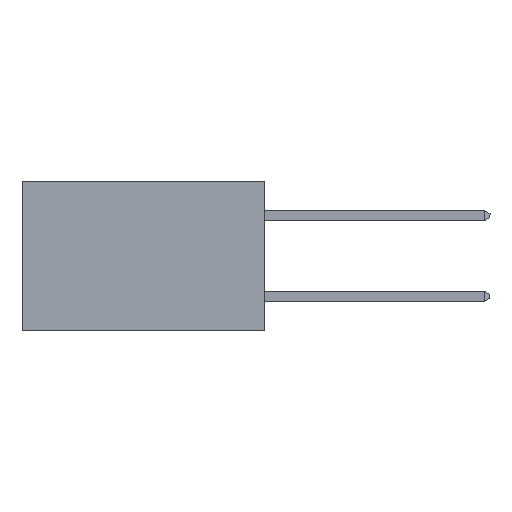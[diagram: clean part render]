
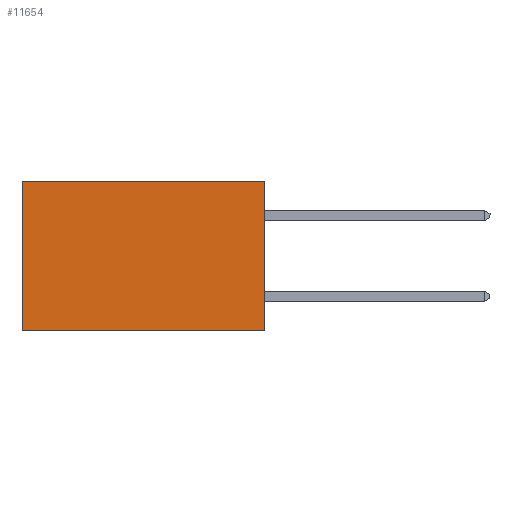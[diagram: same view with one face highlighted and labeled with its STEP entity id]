
A CAD part, left-side view. The second image highlights one B-rep face of the part: STEP entity #11654.
In plain terms, the highlighted planar face has unit normal (-1, 0, 0).
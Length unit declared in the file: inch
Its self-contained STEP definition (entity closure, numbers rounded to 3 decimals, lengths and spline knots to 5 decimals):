
#130 = VERTEX_POINT ( 'NONE', #22287 ) ;
#196 = EDGE_CURVE ( 'NONE', #16527, #12495, #24944, .T. ) ;
#227 = LINE ( 'NONE', #11771, #22972 ) ;
#297 = CARTESIAN_POINT ( 'NONE',  ( 0.298, 0., 0. ) ) ;
#845 = CARTESIAN_POINT ( 'NONE',  ( 0.298, 0., 0. ) ) ;
#877 = DIRECTION ( 'NONE',  ( 0., 1., 0. ) ) ;
#1492 = VERTEX_POINT ( 'NONE', #12076 ) ;
#1498 = CARTESIAN_POINT ( 'NONE',  ( 0.298, 0.6, 0. ) ) ;
#3010 = CARTESIAN_POINT ( 'NONE',  ( 0.298, 0., -0.37 ) ) ;
#4934 = EDGE_CURVE ( 'NONE', #12495, #1492, #24356, .T. ) ;
#4950 = EDGE_CURVE ( 'NONE', #16527, #130, #227, .T. ) ;
#7619 = ORIENTED_EDGE ( 'NONE', *, *, #4950, .F. ) ;
#8640 = ORIENTED_EDGE ( 'NONE', *, *, #10909, .F. ) ;
#8860 = ORIENTED_EDGE ( 'NONE', *, *, #4934, .T. ) ;
#8890 = EDGE_LOOP ( 'NONE', ( #8860, #8640, #7619, #25850 ) ) ;
#9724 = DIRECTION ( 'NONE',  ( 1., 0., 0. ) ) ;
#10909 = EDGE_CURVE ( 'NONE', #130, #1492, #22131, .T. ) ;
#11423 = DIRECTION ( 'NONE',  ( 0., 0., -1. ) ) ;
#11654 = ADVANCED_FACE ( 'NONE', ( #19253 ), #22913, .F. ) ;
#11771 = CARTESIAN_POINT ( 'NONE',  ( 0.298, 0., 0. ) ) ;
#11801 = CARTESIAN_POINT ( 'NONE',  ( 0.298, 0.6, 0. ) ) ;
#12076 = CARTESIAN_POINT ( 'NONE',  ( 0.298, 0.6, -0.37 ) ) ;
#12426 = DIRECTION ( 'NONE',  ( 0., 0., -1. ) ) ;
#12495 = VERTEX_POINT ( 'NONE', #1498 ) ;
#14396 = CARTESIAN_POINT ( 'NONE',  ( 0.298, 0., 0. ) ) ;
#16245 = VECTOR ( 'NONE', #877, 39.37008 ) ;
#16527 = VERTEX_POINT ( 'NONE', #297 ) ;
#17837 = VECTOR ( 'NONE', #11423, 39.37008 ) ;
#19100 = VECTOR ( 'NONE', #22824, 39.37008 ) ;
#19253 = FACE_OUTER_BOUND ( 'NONE', #8890, .T. ) ;
#22131 = LINE ( 'NONE', #3010, #16245 ) ;
#22287 = CARTESIAN_POINT ( 'NONE',  ( 0.298, 0., -0.37 ) ) ;
#22824 = DIRECTION ( 'NONE',  ( 0., 1., 0. ) ) ;
#22913 = PLANE ( 'NONE',  #27165 ) ;
#22972 = VECTOR ( 'NONE', #12426, 39.37008 ) ;
#24356 = LINE ( 'NONE', #11801, #17837 ) ;
#24944 = LINE ( 'NONE', #14396, #19100 ) ;
#25105 = DIRECTION ( 'NONE',  ( 0., 0., -1. ) ) ;
#25850 = ORIENTED_EDGE ( 'NONE', *, *, #196, .T. ) ;
#27165 = AXIS2_PLACEMENT_3D ( 'NONE', #845, #9724, #25105 ) ;
